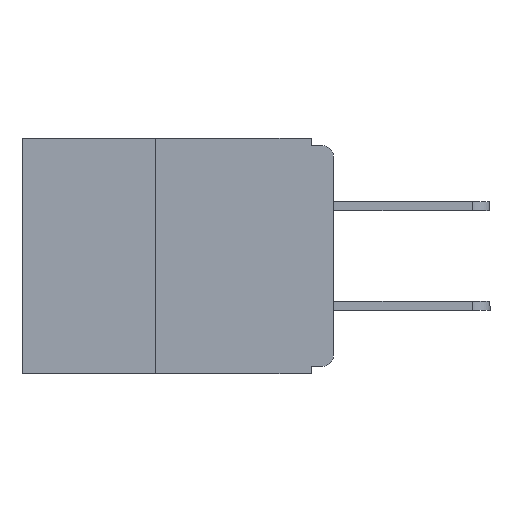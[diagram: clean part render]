
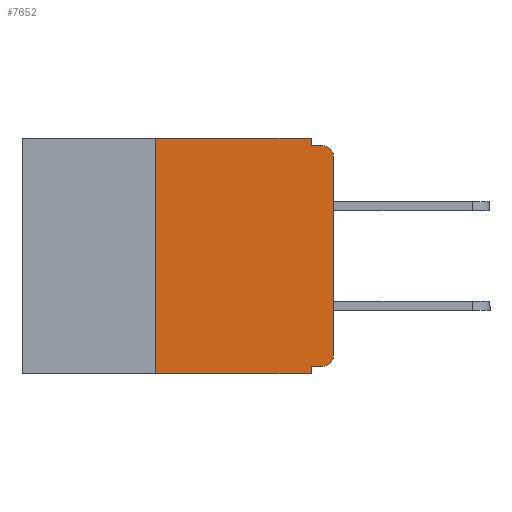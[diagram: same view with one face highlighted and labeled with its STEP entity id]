
A CAD part, left-side view. The second image highlights one B-rep face of the part: STEP entity #7652.
In plain terms, the highlighted planar face has unit normal (-1, 0, 0).
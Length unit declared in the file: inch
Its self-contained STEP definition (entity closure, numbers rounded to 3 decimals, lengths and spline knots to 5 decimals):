
#395 = VERTEX_POINT ( 'NONE', #10389 ) ;
#448 = EDGE_CURVE ( 'NONE', #12003, #9330, #19697, .T. ) ;
#646 = ORIENTED_EDGE ( 'NONE', *, *, #18321, .F. ) ;
#1014 = CARTESIAN_POINT ( 'NONE',  ( 0., 0.437, 0. ) ) ;
#1685 = EDGE_CURVE ( 'NONE', #13244, #14548, #8598, .T. ) ;
#2137 = EDGE_CURVE ( 'NONE', #395, #14548, #22568, .T. ) ;
#2854 = AXIS2_PLACEMENT_3D ( 'NONE', #19910, #8483, #21802 ) ;
#3090 = ORIENTED_EDGE ( 'NONE', *, *, #2137, .F. ) ;
#3742 = LINE ( 'NONE', #1014, #13681 ) ;
#3926 = FACE_OUTER_BOUND ( 'NONE', #20705, .T. ) ;
#4237 = ORIENTED_EDGE ( 'NONE', *, *, #14391, .T. ) ;
#4279 = VECTOR ( 'NONE', #10654, 39.37008 ) ;
#4771 = AXIS2_PLACEMENT_3D ( 'NONE', #16559, #18445, #6944 ) ;
#5210 = ORIENTED_EDGE ( 'NONE', *, *, #19811, .T. ) ;
#6217 = ORIENTED_EDGE ( 'NONE', *, *, #1685, .T. ) ;
#6278 = CARTESIAN_POINT ( 'NONE',  ( 0., 0.031, -0.33 ) ) ;
#6731 = VERTEX_POINT ( 'NONE', #19486 ) ;
#6939 = ORIENTED_EDGE ( 'NONE', *, *, #448, .F. ) ;
#6944 = DIRECTION ( 'NONE',  ( 0., 0., -1. ) ) ;
#7652 = ADVANCED_FACE ( 'NONE', ( #3926 ), #10884, .F. ) ;
#7694 = VERTEX_POINT ( 'NONE', #20519 ) ;
#7745 = VECTOR ( 'NONE', #18484, 39.37008 ) ;
#7754 = DIRECTION ( 'NONE',  ( 0., -1., 0. ) ) ;
#7769 = VERTEX_POINT ( 'NONE', #20671 ) ;
#7798 = LINE ( 'NONE', #24054, #13069 ) ;
#7846 = CARTESIAN_POINT ( 'NONE',  ( 0., 0., -0.01 ) ) ;
#7934 = VECTOR ( 'NONE', #7754, 39.37008 ) ;
#8447 = LINE ( 'NONE', #24838, #18030 ) ;
#8483 = DIRECTION ( 'NONE',  ( -1., 0., 0. ) ) ;
#8598 = CIRCLE ( 'NONE', #24621, 0.015 ) ;
#8976 = DIRECTION ( 'NONE',  ( 0., 0., -1. ) ) ;
#9322 = ORIENTED_EDGE ( 'NONE', *, *, #13993, .F. ) ;
#9330 = VERTEX_POINT ( 'NONE', #10172 ) ;
#9787 = DIRECTION ( 'NONE',  ( 0., 0., -1. ) ) ;
#10172 = CARTESIAN_POINT ( 'NONE',  ( 0., 0.031, -0.33 ) ) ;
#10209 = VECTOR ( 'NONE', #9787, 39.37008 ) ;
#10233 = VERTEX_POINT ( 'NONE', #13909 ) ;
#10389 = CARTESIAN_POINT ( 'NONE',  ( 0., 0.031, -0.01 ) ) ;
#10654 = DIRECTION ( 'NONE',  ( 0., 0., 1. ) ) ;
#10884 = PLANE ( 'NONE',  #4771 ) ;
#11001 = VERTEX_POINT ( 'NONE', #17886 ) ;
#11510 = ORIENTED_EDGE ( 'NONE', *, *, #24848, .F. ) ;
#11601 = ORIENTED_EDGE ( 'NONE', *, *, #14079, .F. ) ;
#11732 = DIRECTION ( 'NONE',  ( 0., 0., 1. ) ) ;
#11904 = CARTESIAN_POINT ( 'NONE',  ( 0., 0.437, -0.33 ) ) ;
#12003 = VERTEX_POINT ( 'NONE', #13754 ) ;
#12058 = DIRECTION ( 'NONE',  ( 0., 0., -1. ) ) ;
#12335 = CARTESIAN_POINT ( 'NONE',  ( 0., 0.015, -0.01 ) ) ;
#12439 = DIRECTION ( 'NONE',  ( -1., 0., 0. ) ) ;
#13069 = VECTOR ( 'NONE', #8976, 39.37008 ) ;
#13244 = VERTEX_POINT ( 'NONE', #15799 ) ;
#13681 = VECTOR ( 'NONE', #18594, 39.37008 ) ;
#13754 = CARTESIAN_POINT ( 'NONE',  ( 0., 0.031, -0.32 ) ) ;
#13909 = CARTESIAN_POINT ( 'NONE',  ( 0., 0.015, -0.32 ) ) ;
#13993 = EDGE_CURVE ( 'NONE', #7694, #7769, #24713, .T. ) ;
#14021 = ORIENTED_EDGE ( 'NONE', *, *, #22810, .T. ) ;
#14079 = EDGE_CURVE ( 'NONE', #10233, #12003, #18540, .T. ) ;
#14391 = EDGE_CURVE ( 'NONE', #7694, #9330, #19715, .T. ) ;
#14548 = VERTEX_POINT ( 'NONE', #12335 ) ;
#15286 = VECTOR ( 'NONE', #24996, 39.37008 ) ;
#15799 = CARTESIAN_POINT ( 'NONE',  ( 0., 0., -0.025 ) ) ;
#16559 = CARTESIAN_POINT ( 'NONE',  ( 0., 0.437, 0. ) ) ;
#16602 = CARTESIAN_POINT ( 'NONE',  ( 0., 0., -0.32 ) ) ;
#17886 = CARTESIAN_POINT ( 'NONE',  ( 0., 0., -0.305 ) ) ;
#18030 = VECTOR ( 'NONE', #11732, 39.37008 ) ;
#18321 = EDGE_CURVE ( 'NONE', #7769, #6731, #3742, .T. ) ;
#18445 = DIRECTION ( 'NONE',  ( 1., 0., 0. ) ) ;
#18484 = DIRECTION ( 'NONE',  ( 0., 1., 0. ) ) ;
#18540 = LINE ( 'NONE', #16602, #7745 ) ;
#18594 = DIRECTION ( 'NONE',  ( 0., -1., 0. ) ) ;
#19486 = CARTESIAN_POINT ( 'NONE',  ( 0., 0.031, 0. ) ) ;
#19697 = LINE ( 'NONE', #6278, #10209 ) ;
#19715 = LINE ( 'NONE', #11904, #15286 ) ;
#19811 = EDGE_CURVE ( 'NONE', #11001, #13244, #8447, .T. ) ;
#19910 = CARTESIAN_POINT ( 'NONE',  ( 0., 0.015, -0.305 ) ) ;
#20075 = CARTESIAN_POINT ( 'NONE',  ( 0., 0.25, -0.33 ) ) ;
#20519 = CARTESIAN_POINT ( 'NONE',  ( 0., 0.25, -0.33 ) ) ;
#20671 = CARTESIAN_POINT ( 'NONE',  ( 0., 0.25, 0. ) ) ;
#20705 = EDGE_LOOP ( 'NONE', ( #5210, #6217, #3090, #11510, #646, #9322, #4237, #6939, #11601, #14021 ) ) ;
#21802 = DIRECTION ( 'NONE',  ( 0., 0., -1. ) ) ;
#22568 = LINE ( 'NONE', #7846, #7934 ) ;
#22810 = EDGE_CURVE ( 'NONE', #10233, #11001, #24360, .T. ) ;
#24054 = CARTESIAN_POINT ( 'NONE',  ( 0., 0.031, 0. ) ) ;
#24336 = CARTESIAN_POINT ( 'NONE',  ( 0., 0.015, -0.025 ) ) ;
#24360 = CIRCLE ( 'NONE', #2854, 0.015 ) ;
#24621 = AXIS2_PLACEMENT_3D ( 'NONE', #24336, #12439, #12058 ) ;
#24713 = LINE ( 'NONE', #20075, #4279 ) ;
#24838 = CARTESIAN_POINT ( 'NONE',  ( 0., 0., 0. ) ) ;
#24848 = EDGE_CURVE ( 'NONE', #6731, #395, #7798, .T. ) ;
#24996 = DIRECTION ( 'NONE',  ( 0., -1., 0. ) ) ;
